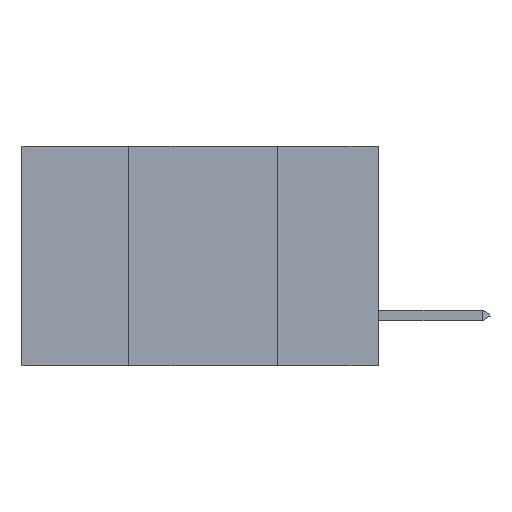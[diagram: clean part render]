
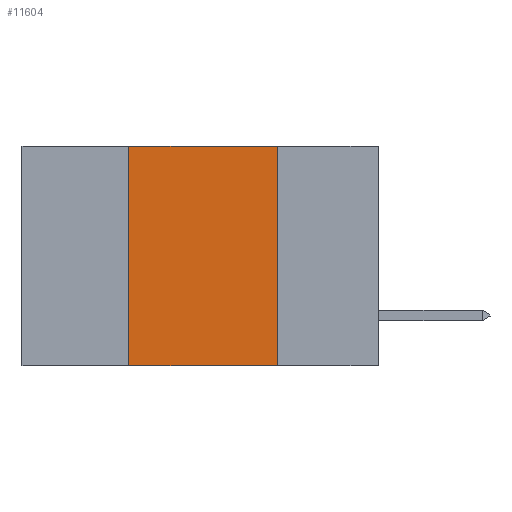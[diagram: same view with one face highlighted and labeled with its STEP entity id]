
A CAD part, left-side view. The second image highlights one B-rep face of the part: STEP entity #11604.
In plain terms, the highlighted planar face has unit normal (-1, 0, 0).
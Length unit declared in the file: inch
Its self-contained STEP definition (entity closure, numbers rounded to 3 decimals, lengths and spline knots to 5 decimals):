
#984 = EDGE_CURVE ( 'NONE', #6563, #12044, #13549, .T. ) ;
#1473 = VERTEX_POINT ( 'NONE', #6533 ) ;
#1733 = CARTESIAN_POINT ( 'NONE',  ( 0., 0.42, 0. ) ) ;
#1984 = CARTESIAN_POINT ( 'NONE',  ( 0., 0.6, 0. ) ) ;
#2018 = VERTEX_POINT ( 'NONE', #4911 ) ;
#3647 = DIRECTION ( 'NONE',  ( 0., 0., -1. ) ) ;
#3695 = ORIENTED_EDGE ( 'NONE', *, *, #984, .F. ) ;
#4512 = VECTOR ( 'NONE', #12450, 39.37008 ) ;
#4643 = CARTESIAN_POINT ( 'NONE',  ( 0., 0.17, 0. ) ) ;
#4911 = CARTESIAN_POINT ( 'NONE',  ( 0., 0.17, -0.37 ) ) ;
#5983 = DIRECTION ( 'NONE',  ( 0., 0., 1. ) ) ;
#6203 = ORIENTED_EDGE ( 'NONE', *, *, #12189, .F. ) ;
#6333 = VECTOR ( 'NONE', #5983, 39.37008 ) ;
#6533 = CARTESIAN_POINT ( 'NONE',  ( 0., 0.42, -0.37 ) ) ;
#6563 = VERTEX_POINT ( 'NONE', #11297 ) ;
#6691 = EDGE_CURVE ( 'NONE', #1473, #2018, #13224, .T. ) ;
#7188 = VECTOR ( 'NONE', #3647, 39.37008 ) ;
#7372 = ORIENTED_EDGE ( 'NONE', *, *, #12817, .F. ) ;
#7523 = FACE_OUTER_BOUND ( 'NONE', #10594, .T. ) ;
#7974 = DIRECTION ( 'NONE',  ( 0., -1., 0. ) ) ;
#8645 = LINE ( 'NONE', #10944, #7188 ) ;
#8971 = DIRECTION ( 'NONE',  ( 0., 0., -1. ) ) ;
#9973 = AXIS2_PLACEMENT_3D ( 'NONE', #10017, #12156, #8971 ) ;
#10017 = CARTESIAN_POINT ( 'NONE',  ( 0., 0.6, 0. ) ) ;
#10594 = EDGE_LOOP ( 'NONE', ( #6203, #3695, #7372, #13477 ) ) ;
#10944 = CARTESIAN_POINT ( 'NONE',  ( 0., 0.17, 0. ) ) ;
#10947 = CARTESIAN_POINT ( 'NONE',  ( 0., 0.6, -0.37 ) ) ;
#11297 = CARTESIAN_POINT ( 'NONE',  ( 0., 0.42, 0. ) ) ;
#11604 = ADVANCED_FACE ( 'NONE', ( #7523 ), #13234, .F. ) ;
#11755 = LINE ( 'NONE', #1733, #6333 ) ;
#12044 = VERTEX_POINT ( 'NONE', #4643 ) ;
#12104 = VECTOR ( 'NONE', #7974, 39.37008 ) ;
#12156 = DIRECTION ( 'NONE',  ( 1., 0., 0. ) ) ;
#12189 = EDGE_CURVE ( 'NONE', #12044, #2018, #8645, .T. ) ;
#12450 = DIRECTION ( 'NONE',  ( 0., -1., 0. ) ) ;
#12817 = EDGE_CURVE ( 'NONE', #1473, #6563, #11755, .T. ) ;
#13224 = LINE ( 'NONE', #10947, #12104 ) ;
#13234 = PLANE ( 'NONE',  #9973 ) ;
#13477 = ORIENTED_EDGE ( 'NONE', *, *, #6691, .T. ) ;
#13549 = LINE ( 'NONE', #1984, #4512 ) ;
